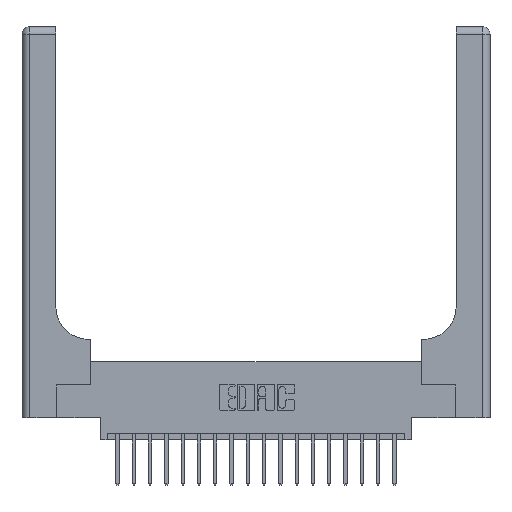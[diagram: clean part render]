
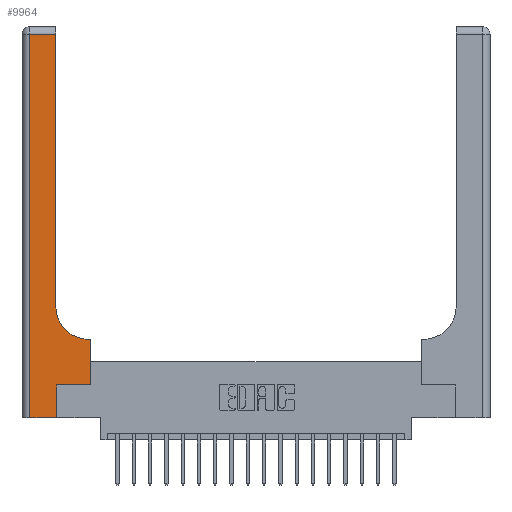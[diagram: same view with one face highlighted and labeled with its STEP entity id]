
A CAD part, top view. The second image highlights one B-rep face of the part: STEP entity #9964.
In plain terms, the highlighted planar face has unit normal (0, 0, 1).
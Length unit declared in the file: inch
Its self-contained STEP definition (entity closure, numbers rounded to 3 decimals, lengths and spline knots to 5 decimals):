
#93 = CARTESIAN_POINT ( 'NONE',  ( 0.51, 0.6, 0.37 ) ) ;
#266 = CARTESIAN_POINT ( 'NONE',  ( 0.265, 0., 0.37 ) ) ;
#304 = LINE ( 'NONE', #9136, #16030 ) ;
#434 = ORIENTED_EDGE ( 'NONE', *, *, #7530, .T. ) ;
#483 = CARTESIAN_POINT ( 'NONE',  ( 0.528, 0.25, 0.37 ) ) ;
#564 = VERTEX_POINT ( 'NONE', #3229 ) ;
#640 = EDGE_CURVE ( 'NONE', #564, #752, #9971, .T. ) ;
#659 = CARTESIAN_POINT ( 'NONE',  ( 0.528, 0.25, 0.37 ) ) ;
#700 = LINE ( 'NONE', #4363, #16426 ) ;
#752 = VERTEX_POINT ( 'NONE', #3645 ) ;
#1944 = VECTOR ( 'NONE', #2083, 39.37008 ) ;
#2083 = DIRECTION ( 'NONE',  ( 0., 1., 0. ) ) ;
#2337 = CARTESIAN_POINT ( 'NONE',  ( 0.06, 0., 0.37 ) ) ;
#3229 = CARTESIAN_POINT ( 'NONE',  ( 0.265, 0., 0.37 ) ) ;
#3541 = CARTESIAN_POINT ( 'NONE',  ( 0.06, 3., 0.37 ) ) ;
#3542 = AXIS2_PLACEMENT_3D ( 'NONE', #9219, #20213, #10790 ) ;
#3559 = VERTEX_POINT ( 'NONE', #11723 ) ;
#3645 = CARTESIAN_POINT ( 'NONE',  ( 0.265, 0.25, 0.37 ) ) ;
#3791 = ORIENTED_EDGE ( 'NONE', *, *, #11067, .T. ) ;
#4253 = VERTEX_POINT ( 'NONE', #2337 ) ;
#4363 = CARTESIAN_POINT ( 'NONE',  ( 0.26, 0.6, 0.37 ) ) ;
#4426 = CARTESIAN_POINT ( 'NONE',  ( 0., 0., 0.37 ) ) ;
#4517 = VECTOR ( 'NONE', #6490, 39.37008 ) ;
#4533 = DIRECTION ( 'NONE',  ( -1., 0., 0. ) ) ;
#4906 = CARTESIAN_POINT ( 'NONE',  ( 0.265, 0.25, 0.37 ) ) ;
#5095 = DIRECTION ( 'NONE',  ( 0., -1., 0. ) ) ;
#5806 = VECTOR ( 'NONE', #14416, 39.37008 ) ;
#6063 = LINE ( 'NONE', #13224, #13924 ) ;
#6353 = ORIENTED_EDGE ( 'NONE', *, *, #11745, .T. ) ;
#6490 = DIRECTION ( 'NONE',  ( 1., 0., 0. ) ) ;
#6618 = ORIENTED_EDGE ( 'NONE', *, *, #6623, .T. ) ;
#6623 = EDGE_CURVE ( 'NONE', #14640, #11235, #700, .T. ) ;
#6697 = VECTOR ( 'NONE', #5095, 39.37008 ) ;
#7530 = EDGE_CURVE ( 'NONE', #15928, #14640, #14468, .T. ) ;
#8113 = EDGE_LOOP ( 'NONE', ( #9859, #16332, #16879, #3791, #14704, #13554, #434, #6618, #6353 ) ) ;
#9086 = DIRECTION ( 'NONE',  ( 1., 0., 0. ) ) ;
#9136 = CARTESIAN_POINT ( 'NONE',  ( 0.26, 3., 0.37 ) ) ;
#9219 = CARTESIAN_POINT ( 'NONE',  ( 0.51, 0.85, 0.37 ) ) ;
#9397 = AXIS2_PLACEMENT_3D ( 'NONE', #18611, #13935, #4533 ) ;
#9859 = ORIENTED_EDGE ( 'NONE', *, *, #14123, .T. ) ;
#9964 = ADVANCED_FACE ( 'NONE', ( #16658 ), #12341, .F. ) ;
#9971 = LINE ( 'NONE', #266, #5806 ) ;
#10393 = EDGE_CURVE ( 'NONE', #20171, #19561, #6063, .T. ) ;
#10439 = LINE ( 'NONE', #4426, #18318 ) ;
#10790 = DIRECTION ( 'NONE',  ( 1., 0., 0. ) ) ;
#11067 = EDGE_CURVE ( 'NONE', #4253, #564, #10439, .T. ) ;
#11235 = VERTEX_POINT ( 'NONE', #93 ) ;
#11723 = CARTESIAN_POINT ( 'NONE',  ( 0.26, 0.85, 0.37 ) ) ;
#11745 = EDGE_CURVE ( 'NONE', #11235, #3559, #18828, .T. ) ;
#12341 = PLANE ( 'NONE',  #9397 ) ;
#13108 = EDGE_CURVE ( 'NONE', #752, #15928, #13352, .T. ) ;
#13224 = CARTESIAN_POINT ( 'NONE',  ( 0., 2.94, 0.37 ) ) ;
#13352 = LINE ( 'NONE', #4906, #4517 ) ;
#13554 = ORIENTED_EDGE ( 'NONE', *, *, #13108, .T. ) ;
#13722 = EDGE_CURVE ( 'NONE', #19561, #4253, #19226, .T. ) ;
#13877 = DIRECTION ( 'NONE',  ( 0., 1., 0. ) ) ;
#13924 = VECTOR ( 'NONE', #14826, 39.37008 ) ;
#13935 = DIRECTION ( 'NONE',  ( 0., 0., -1. ) ) ;
#14123 = EDGE_CURVE ( 'NONE', #3559, #20171, #304, .T. ) ;
#14416 = DIRECTION ( 'NONE',  ( 0., 1., 0. ) ) ;
#14468 = LINE ( 'NONE', #483, #1944 ) ;
#14640 = VERTEX_POINT ( 'NONE', #18777 ) ;
#14704 = ORIENTED_EDGE ( 'NONE', *, *, #640, .T. ) ;
#14826 = DIRECTION ( 'NONE',  ( -1., 0., 0. ) ) ;
#15561 = CARTESIAN_POINT ( 'NONE',  ( 0.06, 2.94, 0.37 ) ) ;
#15928 = VERTEX_POINT ( 'NONE', #659 ) ;
#16030 = VECTOR ( 'NONE', #13877, 39.37008 ) ;
#16332 = ORIENTED_EDGE ( 'NONE', *, *, #10393, .T. ) ;
#16426 = VECTOR ( 'NONE', #20086, 39.37008 ) ;
#16658 = FACE_OUTER_BOUND ( 'NONE', #8113, .T. ) ;
#16879 = ORIENTED_EDGE ( 'NONE', *, *, #13722, .T. ) ;
#18318 = VECTOR ( 'NONE', #9086, 39.37008 ) ;
#18611 = CARTESIAN_POINT ( 'NONE',  ( 0., 3., 0.37 ) ) ;
#18777 = CARTESIAN_POINT ( 'NONE',  ( 0.528, 0.6, 0.37 ) ) ;
#18828 = CIRCLE ( 'NONE', #3542, 0.25 ) ;
#19226 = LINE ( 'NONE', #3541, #6697 ) ;
#19561 = VERTEX_POINT ( 'NONE', #15561 ) ;
#19616 = CARTESIAN_POINT ( 'NONE',  ( 0.26, 2.94, 0.37 ) ) ;
#20086 = DIRECTION ( 'NONE',  ( -1., 0., 0. ) ) ;
#20171 = VERTEX_POINT ( 'NONE', #19616 ) ;
#20213 = DIRECTION ( 'NONE',  ( 0., 0., -1. ) ) ;
